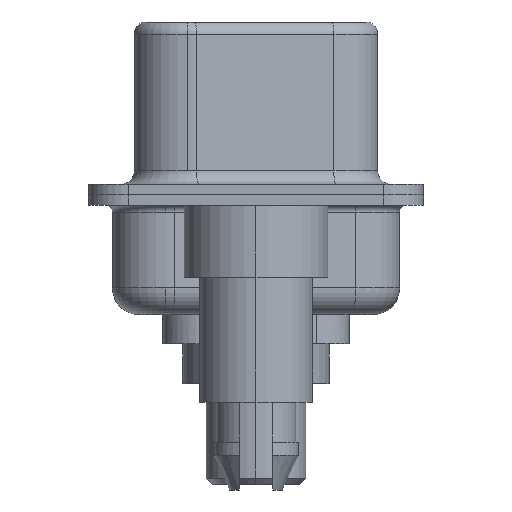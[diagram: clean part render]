
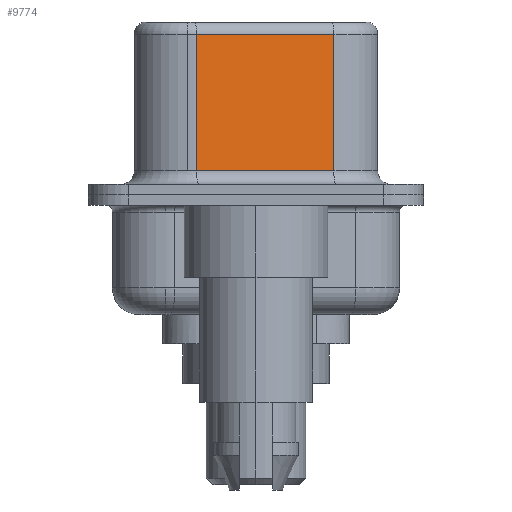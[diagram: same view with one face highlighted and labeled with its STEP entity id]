
A CAD part, left-side view. The second image highlights one B-rep face of the part: STEP entity #9774.
In plain terms, the highlighted planar face has unit normal (-0.985, -0.174, 0).
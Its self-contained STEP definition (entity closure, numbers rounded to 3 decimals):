
#554 = VERTEX_POINT ( 'NONE', #9859 ) ;
#708 = VECTOR ( 'NONE', #2927, 1000. ) ;
#2543 = CARTESIAN_POINT ( 'NONE',  ( 3.67, 2.233, 6.52 ) ) ;
#2621 = AXIS2_PLACEMENT_3D ( 'NONE', #2696, #14569, #5686 ) ;
#2696 = CARTESIAN_POINT ( 'NONE',  ( 4.58, -2.927, 6.52 ) ) ;
#2927 = DIRECTION ( 'NONE',  ( -0.174, 0.985, 0. ) ) ;
#4003 = EDGE_LOOP ( 'NONE', ( #10293, #12345, #9138, #12265 ) ) ;
#4069 = DIRECTION ( 'NONE',  ( 0., 0., -1. ) ) ;
#4274 = EDGE_CURVE ( 'NONE', #9793, #15300, #10769, .T. ) ;
#4435 = EDGE_CURVE ( 'NONE', #4738, #15300, #8873, .T. ) ;
#4678 = LINE ( 'NONE', #7237, #708 ) ;
#4738 = VERTEX_POINT ( 'NONE', #14046 ) ;
#5081 = VECTOR ( 'NONE', #5831, 1000. ) ;
#5686 = DIRECTION ( 'NONE',  ( -0.174, 0.985, 0. ) ) ;
#5831 = DIRECTION ( 'NONE',  ( 0.174, -0.985, 0. ) ) ;
#6095 = FACE_OUTER_BOUND ( 'NONE', #4003, .T. ) ;
#6855 = VECTOR ( 'NONE', #17945, 1000. ) ;
#7237 = CARTESIAN_POINT ( 'NONE',  ( 4.58, -2.927, 6.02 ) ) ;
#8063 = VECTOR ( 'NONE', #4069, 1000. ) ;
#8534 = CARTESIAN_POINT ( 'NONE',  ( 4.58, -2.927, 6.02 ) ) ;
#8693 = CARTESIAN_POINT ( 'NONE',  ( 4.58, -2.927, 0.9 ) ) ;
#8873 = LINE ( 'NONE', #8693, #5081 ) ;
#9138 = ORIENTED_EDGE ( 'NONE', *, *, #10352, .T. ) ;
#9774 = ADVANCED_FACE ( 'NONE', ( #6095 ), #9925, .F. ) ;
#9793 = VERTEX_POINT ( 'NONE', #8534 ) ;
#9859 = CARTESIAN_POINT ( 'NONE',  ( 3.67, 2.233, 6.02 ) ) ;
#9925 = PLANE ( 'NONE',  #2621 ) ;
#10293 = ORIENTED_EDGE ( 'NONE', *, *, #4274, .F. ) ;
#10352 = EDGE_CURVE ( 'NONE', #554, #4738, #16526, .T. ) ;
#10769 = LINE ( 'NONE', #12675, #6855 ) ;
#12204 = EDGE_CURVE ( 'NONE', #9793, #554, #4678, .T. ) ;
#12265 = ORIENTED_EDGE ( 'NONE', *, *, #4435, .T. ) ;
#12345 = ORIENTED_EDGE ( 'NONE', *, *, #12204, .T. ) ;
#12675 = CARTESIAN_POINT ( 'NONE',  ( 4.58, -2.927, 6.52 ) ) ;
#14046 = CARTESIAN_POINT ( 'NONE',  ( 3.67, 2.233, 0.9 ) ) ;
#14569 = DIRECTION ( 'NONE',  ( 0.985, 0.174, 0. ) ) ;
#14926 = CARTESIAN_POINT ( 'NONE',  ( 4.58, -2.927, 0.9 ) ) ;
#15300 = VERTEX_POINT ( 'NONE', #14926 ) ;
#16526 = LINE ( 'NONE', #2543, #8063 ) ;
#17945 = DIRECTION ( 'NONE',  ( 0., 0., -1. ) ) ;
